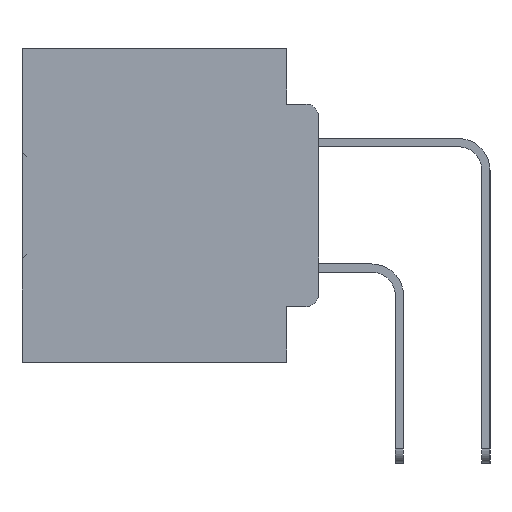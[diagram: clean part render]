
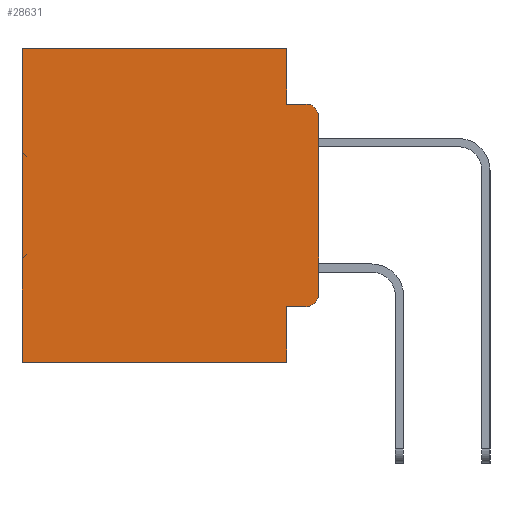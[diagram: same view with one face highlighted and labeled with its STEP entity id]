
A CAD part, left-side view. The second image highlights one B-rep face of the part: STEP entity #28631.
In plain terms, the highlighted planar face has unit normal (-1, 0, 0).
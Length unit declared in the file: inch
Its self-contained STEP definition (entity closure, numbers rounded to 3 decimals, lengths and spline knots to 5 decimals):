
#552 = EDGE_CURVE ( 'NONE', #13873, #25081, #732, .T. ) ;
#732 = LINE ( 'NONE', #2988, #23552 ) ;
#755 = LINE ( 'NONE', #5574, #7958 ) ;
#1567 = CARTESIAN_POINT ( 'NONE',  ( 0.298, 0., -0.5 ) ) ;
#1725 = CARTESIAN_POINT ( 'NONE',  ( 0.298, 0.051, -0.4115 ) ) ;
#2622 = CARTESIAN_POINT ( 'NONE',  ( 0.298, 0.051, -0.0885 ) ) ;
#2988 = CARTESIAN_POINT ( 'NONE',  ( 0.298, 0., 0. ) ) ;
#3681 = LINE ( 'NONE', #7749, #18593 ) ;
#4028 = VECTOR ( 'NONE', #32755, 39.37008 ) ;
#4456 = VERTEX_POINT ( 'NONE', #22080 ) ;
#4504 = VERTEX_POINT ( 'NONE', #25097 ) ;
#4613 = ORIENTED_EDGE ( 'NONE', *, *, #552, .F. ) ;
#5574 = CARTESIAN_POINT ( 'NONE',  ( 0.298, 0.473, 0. ) ) ;
#7278 = EDGE_CURVE ( 'NONE', #4456, #12960, #37940, .T. ) ;
#7475 = ORIENTED_EDGE ( 'NONE', *, *, #34838, .T. ) ;
#7503 = EDGE_CURVE ( 'NONE', #4504, #12960, #755, .T. ) ;
#7749 = CARTESIAN_POINT ( 'NONE',  ( 0.298, 0.051, 0. ) ) ;
#7958 = VECTOR ( 'NONE', #14629, 39.37008 ) ;
#9066 = EDGE_CURVE ( 'NONE', #19624, #4504, #19853, .T. ) ;
#9315 = AXIS2_PLACEMENT_3D ( 'NONE', #30088, #12726, #32976 ) ;
#10287 = EDGE_CURVE ( 'NONE', #34892, #25081, #18386, .T. ) ;
#10623 = CARTESIAN_POINT ( 'NONE',  ( 0.298, 0.051, -0.0885 ) ) ;
#10776 = DIRECTION ( 'NONE',  ( 0., 0., -1. ) ) ;
#11253 = ORIENTED_EDGE ( 'NONE', *, *, #9066, .T. ) ;
#11344 = CARTESIAN_POINT ( 'NONE',  ( 0.298, 0.473, -0.5 ) ) ;
#11390 = AXIS2_PLACEMENT_3D ( 'NONE', #29779, #12408, #32661 ) ;
#12187 = FACE_OUTER_BOUND ( 'NONE', #37985, .T. ) ;
#12253 = EDGE_CURVE ( 'NONE', #13357, #34892, #28134, .T. ) ;
#12408 = DIRECTION ( 'NONE',  ( -1., 0., 0. ) ) ;
#12726 = DIRECTION ( 'NONE',  ( 1., 0., 0. ) ) ;
#12960 = VERTEX_POINT ( 'NONE', #11344 ) ;
#13357 = VERTEX_POINT ( 'NONE', #1725 ) ;
#13365 = LINE ( 'NONE', #31289, #34634 ) ;
#13873 = VERTEX_POINT ( 'NONE', #33319 ) ;
#14629 = DIRECTION ( 'NONE',  ( 0., 0., -1. ) ) ;
#15253 = LINE ( 'NONE', #2622, #29699 ) ;
#17787 = DIRECTION ( 'NONE',  ( -1., 0., 0. ) ) ;
#18147 = EDGE_CURVE ( 'NONE', #13357, #4456, #13365, .T. ) ;
#18386 = CIRCLE ( 'NONE', #11390, 0.02 ) ;
#18593 = VECTOR ( 'NONE', #10776, 39.37008 ) ;
#19590 = VECTOR ( 'NONE', #37212, 39.37008 ) ;
#19624 = VERTEX_POINT ( 'NONE', #31929 ) ;
#19853 = LINE ( 'NONE', #29864, #4028 ) ;
#19994 = ORIENTED_EDGE ( 'NONE', *, *, #12253, .T. ) ;
#20151 = VERTEX_POINT ( 'NONE', #20865 ) ;
#20226 = CARTESIAN_POINT ( 'NONE',  ( 0.298, 0., -0.3915 ) ) ;
#20635 = AXIS2_PLACEMENT_3D ( 'NONE', #35080, #17787, #37965 ) ;
#20865 = CARTESIAN_POINT ( 'NONE',  ( 0.298, 0.02, -0.0885 ) ) ;
#22080 = CARTESIAN_POINT ( 'NONE',  ( 0.298, 0.051, -0.5 ) ) ;
#22645 = VECTOR ( 'NONE', #28137, 39.37008 ) ;
#23103 = ORIENTED_EDGE ( 'NONE', *, *, #30989, .F. ) ;
#23552 = VECTOR ( 'NONE', #24576, 39.37008 ) ;
#24576 = DIRECTION ( 'NONE',  ( 0., 0., -1. ) ) ;
#25081 = VERTEX_POINT ( 'NONE', #20226 ) ;
#25097 = CARTESIAN_POINT ( 'NONE',  ( 0.298, 0.473, 0. ) ) ;
#25185 = EDGE_CURVE ( 'NONE', #19624, #32152, #3681, .T. ) ;
#25375 = ORIENTED_EDGE ( 'NONE', *, *, #7503, .T. ) ;
#25760 = CARTESIAN_POINT ( 'NONE',  ( 0.298, 0.051, -0.4115 ) ) ;
#26262 = DIRECTION ( 'NONE',  ( 0., -1., 0. ) ) ;
#26748 = CARTESIAN_POINT ( 'NONE',  ( 0.298, 0.02, -0.4115 ) ) ;
#27902 = CIRCLE ( 'NONE', #20635, 0.02 ) ;
#28134 = LINE ( 'NONE', #25760, #19590 ) ;
#28137 = DIRECTION ( 'NONE',  ( 0., 1., 0. ) ) ;
#28631 = ADVANCED_FACE ( 'NONE', ( #12187 ), #35750, .F. ) ;
#29699 = VECTOR ( 'NONE', #26262, 39.37008 ) ;
#29779 = CARTESIAN_POINT ( 'NONE',  ( 0.298, 0.02, -0.3915 ) ) ;
#29864 = CARTESIAN_POINT ( 'NONE',  ( 0.298, 0., 0. ) ) ;
#30088 = CARTESIAN_POINT ( 'NONE',  ( 0.298, 0., 0. ) ) ;
#30989 = EDGE_CURVE ( 'NONE', #32152, #20151, #15253, .T. ) ;
#31289 = CARTESIAN_POINT ( 'NONE',  ( 0.298, 0.051, 0. ) ) ;
#31929 = CARTESIAN_POINT ( 'NONE',  ( 0.298, 0.051, 0. ) ) ;
#32152 = VERTEX_POINT ( 'NONE', #10623 ) ;
#32661 = DIRECTION ( 'NONE',  ( 0., 0., -1. ) ) ;
#32755 = DIRECTION ( 'NONE',  ( 0., 1., 0. ) ) ;
#32976 = DIRECTION ( 'NONE',  ( 0., 0., -1. ) ) ;
#33022 = ORIENTED_EDGE ( 'NONE', *, *, #7278, .F. ) ;
#33319 = CARTESIAN_POINT ( 'NONE',  ( 0.298, 0., -0.1085 ) ) ;
#33455 = ORIENTED_EDGE ( 'NONE', *, *, #25185, .F. ) ;
#34196 = DIRECTION ( 'NONE',  ( 0., 0., -1. ) ) ;
#34634 = VECTOR ( 'NONE', #34196, 39.37008 ) ;
#34838 = EDGE_CURVE ( 'NONE', #13873, #20151, #27902, .T. ) ;
#34844 = ORIENTED_EDGE ( 'NONE', *, *, #18147, .F. ) ;
#34892 = VERTEX_POINT ( 'NONE', #26748 ) ;
#35080 = CARTESIAN_POINT ( 'NONE',  ( 0.298, 0.02, -0.1085 ) ) ;
#35750 = PLANE ( 'NONE',  #9315 ) ;
#37116 = ORIENTED_EDGE ( 'NONE', *, *, #10287, .T. ) ;
#37212 = DIRECTION ( 'NONE',  ( 0., -1., 0. ) ) ;
#37940 = LINE ( 'NONE', #1567, #22645 ) ;
#37965 = DIRECTION ( 'NONE',  ( 0., 0., -1. ) ) ;
#37985 = EDGE_LOOP ( 'NONE', ( #4613, #7475, #23103, #33455, #11253, #25375, #33022, #34844, #19994, #37116 ) ) ;
